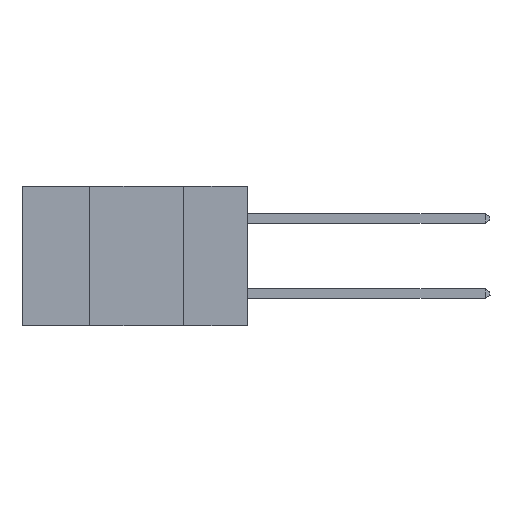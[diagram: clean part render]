
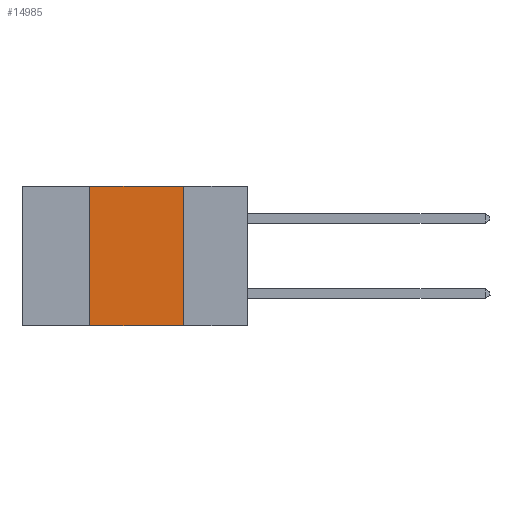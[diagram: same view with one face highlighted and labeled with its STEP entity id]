
A CAD part, left-side view. The second image highlights one B-rep face of the part: STEP entity #14985.
In plain terms, the highlighted planar face has unit normal (-1, 0, 0).
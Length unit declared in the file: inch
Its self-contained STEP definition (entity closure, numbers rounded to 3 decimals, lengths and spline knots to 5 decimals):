
#136 = VERTEX_POINT ( 'NONE', #16425 ) ;
#694 = CARTESIAN_POINT ( 'NONE',  ( 0., 0.42, 0. ) ) ;
#1594 = CARTESIAN_POINT ( 'NONE',  ( 0., 0.6, -0.37 ) ) ;
#1843 = EDGE_CURVE ( 'NONE', #136, #18591, #25236, .T. ) ;
#2488 = DIRECTION ( 'NONE',  ( 0., -1., 0. ) ) ;
#2741 = DIRECTION ( 'NONE',  ( 0., 0., 1. ) ) ;
#3064 = DIRECTION ( 'NONE',  ( 0., -1., 0. ) ) ;
#3429 = VECTOR ( 'NONE', #2741, 39.37008 ) ;
#4323 = ORIENTED_EDGE ( 'NONE', *, *, #11953, .F. ) ;
#4749 = AXIS2_PLACEMENT_3D ( 'NONE', #11574, #25584, #5567 ) ;
#5370 = CARTESIAN_POINT ( 'NONE',  ( 0., 0.6, 0. ) ) ;
#5567 = DIRECTION ( 'NONE',  ( 0., 0., -1. ) ) ;
#6399 = CARTESIAN_POINT ( 'NONE',  ( 0., 0.42, 0. ) ) ;
#6688 = VERTEX_POINT ( 'NONE', #6399 ) ;
#7452 = PLANE ( 'NONE',  #4749 ) ;
#8793 = CARTESIAN_POINT ( 'NONE',  ( 0., 0.17, -0.37 ) ) ;
#9219 = CARTESIAN_POINT ( 'NONE',  ( 0., 0.17, 0. ) ) ;
#9490 = ORIENTED_EDGE ( 'NONE', *, *, #12775, .F. ) ;
#9568 = LINE ( 'NONE', #5370, #20633 ) ;
#11574 = CARTESIAN_POINT ( 'NONE',  ( 0., 0.6, 0. ) ) ;
#11805 = FACE_OUTER_BOUND ( 'NONE', #23537, .T. ) ;
#11953 = EDGE_CURVE ( 'NONE', #6688, #12539, #9568, .T. ) ;
#12342 = ORIENTED_EDGE ( 'NONE', *, *, #1843, .T. ) ;
#12539 = VERTEX_POINT ( 'NONE', #22401 ) ;
#12775 = EDGE_CURVE ( 'NONE', #12539, #18591, #18042, .T. ) ;
#14189 = LINE ( 'NONE', #694, #3429 ) ;
#14985 = ADVANCED_FACE ( 'NONE', ( #11805 ), #7452, .F. ) ;
#16425 = CARTESIAN_POINT ( 'NONE',  ( 0., 0.42, -0.37 ) ) ;
#17402 = DIRECTION ( 'NONE',  ( 0., 0., -1. ) ) ;
#18042 = LINE ( 'NONE', #9219, #25686 ) ;
#18591 = VERTEX_POINT ( 'NONE', #8793 ) ;
#18623 = ORIENTED_EDGE ( 'NONE', *, *, #26033, .F. ) ;
#19796 = VECTOR ( 'NONE', #2488, 39.37008 ) ;
#20633 = VECTOR ( 'NONE', #3064, 39.37008 ) ;
#22401 = CARTESIAN_POINT ( 'NONE',  ( 0., 0.17, 0. ) ) ;
#23537 = EDGE_LOOP ( 'NONE', ( #9490, #4323, #18623, #12342 ) ) ;
#25236 = LINE ( 'NONE', #1594, #19796 ) ;
#25584 = DIRECTION ( 'NONE',  ( 1., 0., 0. ) ) ;
#25686 = VECTOR ( 'NONE', #17402, 39.37008 ) ;
#26033 = EDGE_CURVE ( 'NONE', #136, #6688, #14189, .T. ) ;
